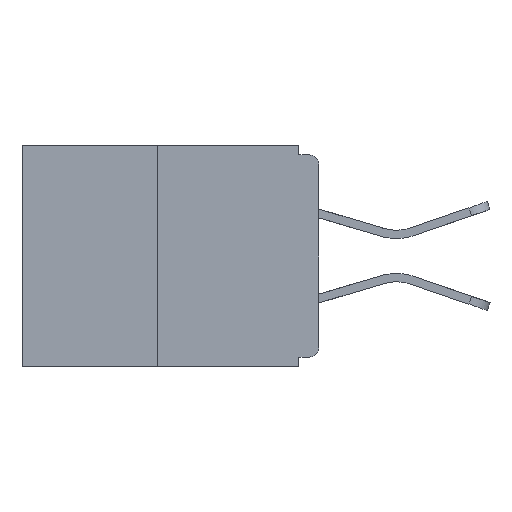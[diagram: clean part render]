
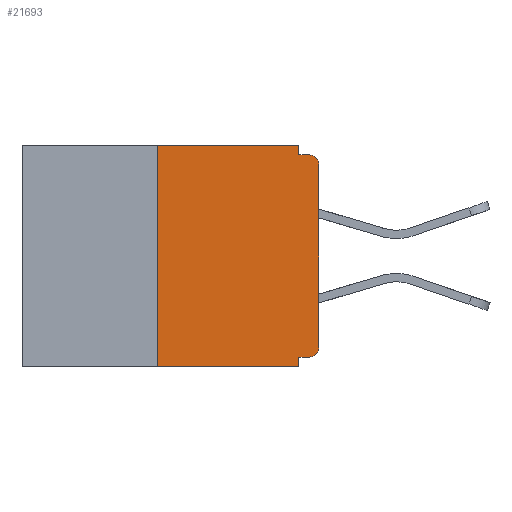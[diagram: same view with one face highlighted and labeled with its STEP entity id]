
A CAD part, left-side view. The second image highlights one B-rep face of the part: STEP entity #21693.
In plain terms, the highlighted planar face has unit normal (-1, 0, 0).
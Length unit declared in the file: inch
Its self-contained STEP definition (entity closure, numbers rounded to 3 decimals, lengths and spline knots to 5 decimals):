
#21 = DIRECTION ( 'NONE',  ( 0., 0., -1. ) ) ;
#938 = DIRECTION ( 'NONE',  ( 0., 0., -1. ) ) ;
#967 = VECTOR ( 'NONE', #18944, 39.37008 ) ;
#1263 = VERTEX_POINT ( 'NONE', #11001 ) ;
#1437 = LINE ( 'NONE', #7302, #16193 ) ;
#1691 = VECTOR ( 'NONE', #4575, 39.37008 ) ;
#2672 = AXIS2_PLACEMENT_3D ( 'NONE', #14578, #6938, #938 ) ;
#2781 = LINE ( 'NONE', #4014, #19682 ) ;
#3780 = CIRCLE ( 'NONE', #2672, 0.015 ) ;
#3952 = LINE ( 'NONE', #7153, #24745 ) ;
#4014 = CARTESIAN_POINT ( 'NONE',  ( 0., 0.25, 0. ) ) ;
#4070 = EDGE_CURVE ( 'NONE', #18503, #7749, #2781, .T. ) ;
#4168 = FACE_OUTER_BOUND ( 'NONE', #8442, .T. ) ;
#4575 = DIRECTION ( 'NONE',  ( 0., 0., -1. ) ) ;
#5256 = EDGE_CURVE ( 'NONE', #18503, #13970, #3952, .T. ) ;
#5613 = VECTOR ( 'NONE', #12287, 39.37008 ) ;
#5957 = DIRECTION ( 'NONE',  ( 0., 0., 1. ) ) ;
#6035 = VERTEX_POINT ( 'NONE', #8571 ) ;
#6087 = LINE ( 'NONE', #7479, #967 ) ;
#6618 = CARTESIAN_POINT ( 'NONE',  ( 0., 0.46, 0. ) ) ;
#6938 = DIRECTION ( 'NONE',  ( -1., 0., 0. ) ) ;
#7020 = ORIENTED_EDGE ( 'NONE', *, *, #19154, .F. ) ;
#7153 = CARTESIAN_POINT ( 'NONE',  ( 0., 0.46, -0.343 ) ) ;
#7251 = EDGE_CURVE ( 'NONE', #21577, #11466, #8377, .T. ) ;
#7302 = CARTESIAN_POINT ( 'NONE',  ( 0., 0., 0. ) ) ;
#7429 = CARTESIAN_POINT ( 'NONE',  ( 0., 0.015, -0.03 ) ) ;
#7479 = CARTESIAN_POINT ( 'NONE',  ( 0., 0.46, 0. ) ) ;
#7560 = ORIENTED_EDGE ( 'NONE', *, *, #5256, .T. ) ;
#7672 = ORIENTED_EDGE ( 'NONE', *, *, #15752, .T. ) ;
#7691 = CARTESIAN_POINT ( 'NONE',  ( 0., 0.031, 0. ) ) ;
#7749 = VERTEX_POINT ( 'NONE', #20703 ) ;
#8377 = CIRCLE ( 'NONE', #23766, 0.015 ) ;
#8410 = CARTESIAN_POINT ( 'NONE',  ( 0., 0.031, 0. ) ) ;
#8442 = EDGE_LOOP ( 'NONE', ( #7020, #11950, #7560, #11463, #12635, #12119, #7672, #24666, #10918, #22874 ) ) ;
#8571 = CARTESIAN_POINT ( 'NONE',  ( 0., 0.031, -0.015 ) ) ;
#8878 = EDGE_CURVE ( 'NONE', #18008, #1263, #24695, .T. ) ;
#9058 = DIRECTION ( 'NONE',  ( 0., -1., 0. ) ) ;
#9337 = CARTESIAN_POINT ( 'NONE',  ( 0., 0.015, -0.015 ) ) ;
#9597 = DIRECTION ( 'NONE',  ( -1., 0., 0. ) ) ;
#10704 = VECTOR ( 'NONE', #23443, 39.37008 ) ;
#10731 = LINE ( 'NONE', #23794, #5613 ) ;
#10738 = CARTESIAN_POINT ( 'NONE',  ( 0., 0., -0.313 ) ) ;
#10918 = ORIENTED_EDGE ( 'NONE', *, *, #22412, .F. ) ;
#11001 = CARTESIAN_POINT ( 'NONE',  ( 0., 0.031, -0.328 ) ) ;
#11064 = DIRECTION ( 'NONE',  ( 0., 0., 1. ) ) ;
#11463 = ORIENTED_EDGE ( 'NONE', *, *, #15575, .F. ) ;
#11466 = VERTEX_POINT ( 'NONE', #9337 ) ;
#11950 = ORIENTED_EDGE ( 'NONE', *, *, #4070, .F. ) ;
#12119 = ORIENTED_EDGE ( 'NONE', *, *, #16392, .T. ) ;
#12287 = DIRECTION ( 'NONE',  ( 0., 0., -1. ) ) ;
#12635 = ORIENTED_EDGE ( 'NONE', *, *, #8878, .F. ) ;
#13970 = VERTEX_POINT ( 'NONE', #20108 ) ;
#14578 = CARTESIAN_POINT ( 'NONE',  ( 0., 0.015, -0.313 ) ) ;
#15575 = EDGE_CURVE ( 'NONE', #1263, #13970, #10731, .T. ) ;
#15752 = EDGE_CURVE ( 'NONE', #23691, #21577, #1437, .T. ) ;
#16193 = VECTOR ( 'NONE', #11064, 39.37008 ) ;
#16392 = EDGE_CURVE ( 'NONE', #18008, #23691, #3780, .T. ) ;
#17096 = LINE ( 'NONE', #8410, #1691 ) ;
#17354 = AXIS2_PLACEMENT_3D ( 'NONE', #6618, #18259, #23952 ) ;
#18008 = VERTEX_POINT ( 'NONE', #20718 ) ;
#18259 = DIRECTION ( 'NONE',  ( 1., 0., 0. ) ) ;
#18503 = VERTEX_POINT ( 'NONE', #24512 ) ;
#18944 = DIRECTION ( 'NONE',  ( 0., -1., 0. ) ) ;
#19154 = EDGE_CURVE ( 'NONE', #7749, #22504, #6087, .T. ) ;
#19161 = DIRECTION ( 'NONE',  ( 0., 1., 0. ) ) ;
#19682 = VECTOR ( 'NONE', #5957, 39.37008 ) ;
#19793 = LINE ( 'NONE', #21265, #10704 ) ;
#20108 = CARTESIAN_POINT ( 'NONE',  ( 0., 0.031, -0.343 ) ) ;
#20703 = CARTESIAN_POINT ( 'NONE',  ( 0., 0.25, 0. ) ) ;
#20718 = CARTESIAN_POINT ( 'NONE',  ( 0., 0.015, -0.328 ) ) ;
#21265 = CARTESIAN_POINT ( 'NONE',  ( 0., 0., -0.015 ) ) ;
#21577 = VERTEX_POINT ( 'NONE', #23324 ) ;
#21693 = ADVANCED_FACE ( 'NONE', ( #4168 ), #23887, .F. ) ;
#22412 = EDGE_CURVE ( 'NONE', #6035, #11466, #19793, .T. ) ;
#22504 = VERTEX_POINT ( 'NONE', #7691 ) ;
#22874 = ORIENTED_EDGE ( 'NONE', *, *, #23650, .F. ) ;
#23324 = CARTESIAN_POINT ( 'NONE',  ( 0., 0., -0.03 ) ) ;
#23443 = DIRECTION ( 'NONE',  ( 0., -1., 0. ) ) ;
#23650 = EDGE_CURVE ( 'NONE', #22504, #6035, #17096, .T. ) ;
#23691 = VERTEX_POINT ( 'NONE', #10738 ) ;
#23766 = AXIS2_PLACEMENT_3D ( 'NONE', #7429, #9597, #21 ) ;
#23794 = CARTESIAN_POINT ( 'NONE',  ( 0., 0.031, -0.343 ) ) ;
#23887 = PLANE ( 'NONE',  #17354 ) ;
#23952 = DIRECTION ( 'NONE',  ( 0., 0., -1. ) ) ;
#24070 = VECTOR ( 'NONE', #19161, 39.37008 ) ;
#24512 = CARTESIAN_POINT ( 'NONE',  ( 0., 0.25, -0.343 ) ) ;
#24666 = ORIENTED_EDGE ( 'NONE', *, *, #7251, .T. ) ;
#24695 = LINE ( 'NONE', #24770, #24070 ) ;
#24745 = VECTOR ( 'NONE', #9058, 39.37008 ) ;
#24770 = CARTESIAN_POINT ( 'NONE',  ( 0., 0., -0.328 ) ) ;
